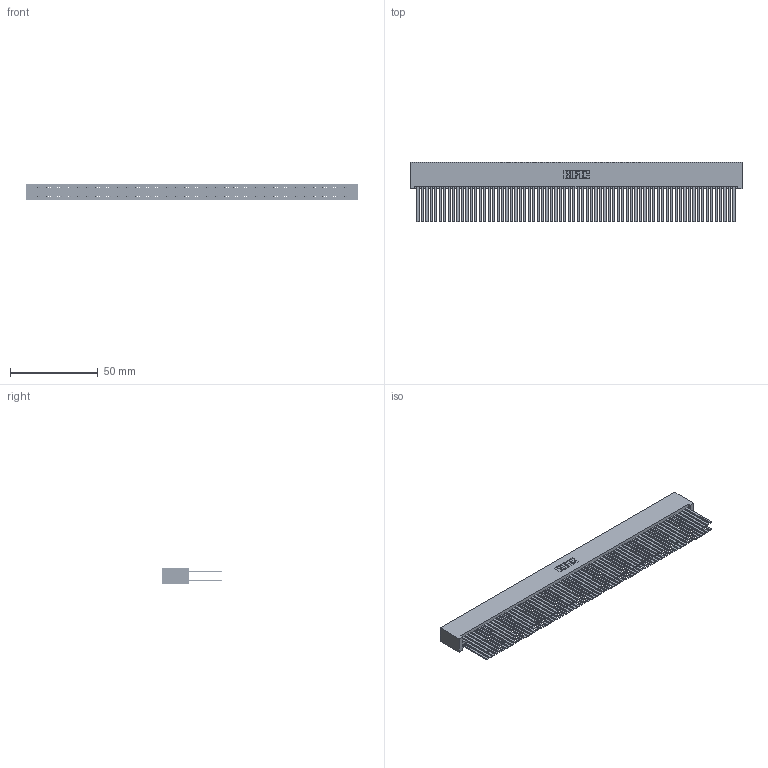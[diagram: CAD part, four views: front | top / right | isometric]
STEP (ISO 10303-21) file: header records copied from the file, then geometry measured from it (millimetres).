
FILE_DESCRIPTION (( 'STEP AP203' ), '1' );
FILE_NAME ('345-144-544-201.STEP', '2019-11-09T10:36:38', ( '' ), ( '' ), 'SwSTEP 2.0', 'SolidWorks 2016', '' );
FILE_SCHEMA (( 'CONFIG_CONTROL_DESIGN' ));
Length unit declared in the file: inch
Products named in the file (3): 345-292-001_345-293-144; 345-144-544-201; 345 Part_No Mounting Lugs
Assembly tree (145 placements, depth 2):
  345-144-544-201
    345 Part_No Mounting Lugs
    345-292-001_345-293-144  x144
Bounding box: 189.48 x 33.96 x 9.4 mm (x, y, z)
Volume: 21319.7 mm3; surface area: 38314.7 mm2
Topology: 145 solids, 145 shells, 6454 faces, 19181 edges, 12594 vertices
Faces by surface type: plane 4252, cylinder 2202
Entity records: 51993 total; most frequent: CARTESIAN_POINT 8684, ORIENTED_EDGE 8618, DIRECTION 7613, EDGE_CURVE 4309, VECTOR 3901, LINE 3901, VERTEX_POINT 2870, AXIS2_PLACEMENT_3D 1856
